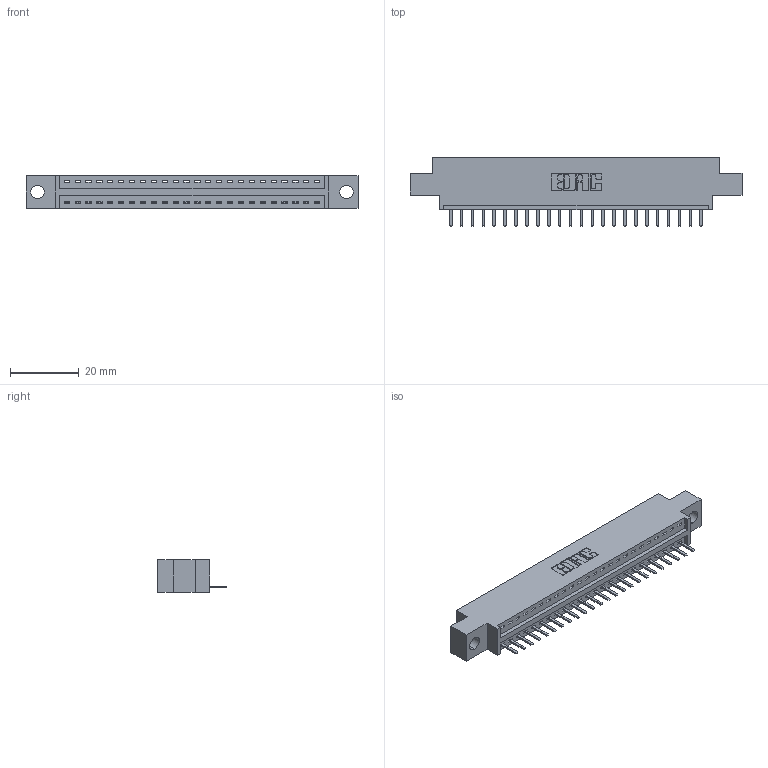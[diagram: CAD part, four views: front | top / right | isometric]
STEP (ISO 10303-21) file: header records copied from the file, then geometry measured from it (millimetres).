
FILE_DESCRIPTION (( 'STEP AP203' ), '1' );
FILE_NAME ('396-024-520-604.STEP', '2019-10-27T05:36:29', ( '' ), ( '' ), 'SwSTEP 2.0', 'SolidWorks 2016', '' );
FILE_SCHEMA (( 'CONFIG_CONTROL_DESIGN' ));
Length unit declared in the file: inch
Products named in the file (3): 396-024-520-604; 346 Part_0.170 Offset - 0.156 Dia-TH; 345-292-001_345-293-120
Assembly tree (25 placements, depth 2):
  396-024-520-604
    346 Part_0.170 Offset - 0.156 Dia-TH
    345-292-001_345-293-120  x24
Bounding box: 96.77 x 20.02 x 9.4 mm (x, y, z)
Volume: 8827.9 mm3; surface area: 10574.3 mm2
Topology: 25 solids, 25 shells, 1614 faces, 4757 edges, 3106 vertices
Faces by surface type: plane 1088, cylinder 526
Entity records: 17567 total; most frequent: CARTESIAN_POINT 3036, ORIENTED_EDGE 2982, DIRECTION 2687, EDGE_CURVE 1491, LINE 1259, VECTOR 1259, VERTEX_POINT 990, AXIS2_PLACEMENT_3D 714
